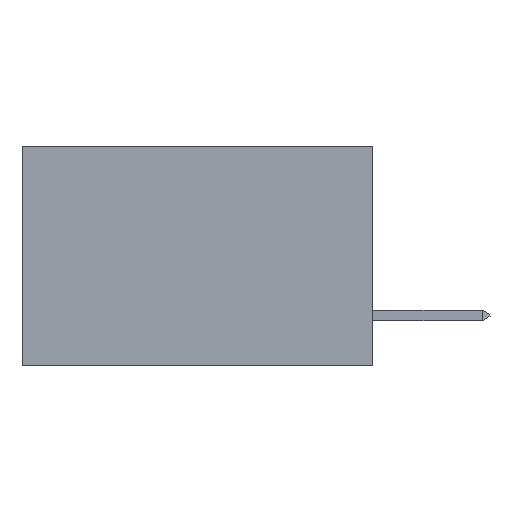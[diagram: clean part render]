
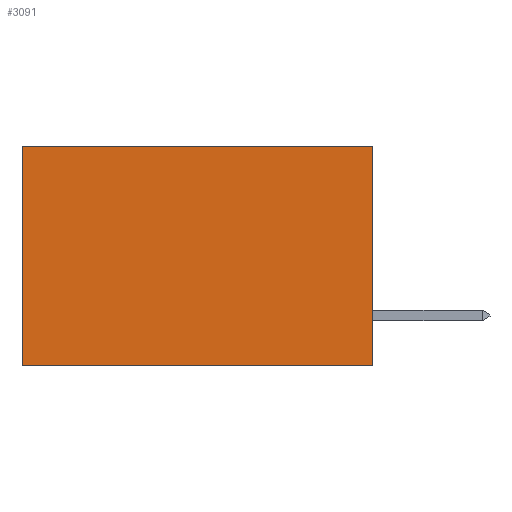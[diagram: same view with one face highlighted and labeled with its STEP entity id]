
A CAD part, left-side view. The second image highlights one B-rep face of the part: STEP entity #3091.
In plain terms, the highlighted planar face has unit normal (-1, 0, 0).
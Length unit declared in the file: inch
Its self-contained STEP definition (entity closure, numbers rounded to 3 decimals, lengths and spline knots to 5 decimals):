
#784 = LINE ( 'NONE', #5822, #5406 ) ;
#1162 = CARTESIAN_POINT ( 'NONE',  ( 0.277, 0.59, -0.37 ) ) ;
#1198 = VECTOR ( 'NONE', #5794, 39.37008 ) ;
#1282 = DIRECTION ( 'NONE',  ( 1., 0., 0. ) ) ;
#2163 = LINE ( 'NONE', #3571, #10662 ) ;
#2646 = VERTEX_POINT ( 'NONE', #6591 ) ;
#3091 = ADVANCED_FACE ( 'NONE', ( #10058 ), #10765, .F. ) ;
#3366 = DIRECTION ( 'NONE',  ( 0., 0., -1. ) ) ;
#3571 = CARTESIAN_POINT ( 'NONE',  ( 0.277, 0., -0.37 ) ) ;
#4044 = CARTESIAN_POINT ( 'NONE',  ( 0.277, 0., 0. ) ) ;
#4071 = AXIS2_PLACEMENT_3D ( 'NONE', #8649, #1282, #8797 ) ;
#4224 = DIRECTION ( 'NONE',  ( 0., 1., 0. ) ) ;
#4536 = VECTOR ( 'NONE', #4224, 39.37008 ) ;
#5002 = ORIENTED_EDGE ( 'NONE', *, *, #6880, .F. ) ;
#5406 = VECTOR ( 'NONE', #7808, 39.37008 ) ;
#5761 = CARTESIAN_POINT ( 'NONE',  ( 0.277, 0., -0.37 ) ) ;
#5794 = DIRECTION ( 'NONE',  ( 0., 1., 0. ) ) ;
#5820 = ORIENTED_EDGE ( 'NONE', *, *, #6698, .F. ) ;
#5822 = CARTESIAN_POINT ( 'NONE',  ( 0.277, 0.59, -0.37 ) ) ;
#6083 = LINE ( 'NONE', #5761, #1198 ) ;
#6435 = CARTESIAN_POINT ( 'NONE',  ( 0.277, 0.59, 0. ) ) ;
#6591 = CARTESIAN_POINT ( 'NONE',  ( 0.277, 0., 0. ) ) ;
#6698 = EDGE_CURVE ( 'NONE', #9893, #7033, #6083, .T. ) ;
#6880 = EDGE_CURVE ( 'NONE', #2646, #9893, #2163, .T. ) ;
#7033 = VERTEX_POINT ( 'NONE', #1162 ) ;
#7314 = ORIENTED_EDGE ( 'NONE', *, *, #7455, .T. ) ;
#7455 = EDGE_CURVE ( 'NONE', #9120, #7033, #784, .T. ) ;
#7808 = DIRECTION ( 'NONE',  ( 0., 0., -1. ) ) ;
#8512 = ORIENTED_EDGE ( 'NONE', *, *, #8717, .T. ) ;
#8649 = CARTESIAN_POINT ( 'NONE',  ( 0.277, 0., -0.37 ) ) ;
#8717 = EDGE_CURVE ( 'NONE', #2646, #9120, #9129, .T. ) ;
#8797 = DIRECTION ( 'NONE',  ( 0., 0., -1. ) ) ;
#8884 = CARTESIAN_POINT ( 'NONE',  ( 0.277, 0., -0.37 ) ) ;
#9120 = VERTEX_POINT ( 'NONE', #6435 ) ;
#9129 = LINE ( 'NONE', #4044, #4536 ) ;
#9893 = VERTEX_POINT ( 'NONE', #8884 ) ;
#10058 = FACE_OUTER_BOUND ( 'NONE', #11028, .T. ) ;
#10662 = VECTOR ( 'NONE', #3366, 39.37008 ) ;
#10765 = PLANE ( 'NONE',  #4071 ) ;
#11028 = EDGE_LOOP ( 'NONE', ( #7314, #5820, #5002, #8512 ) ) ;
